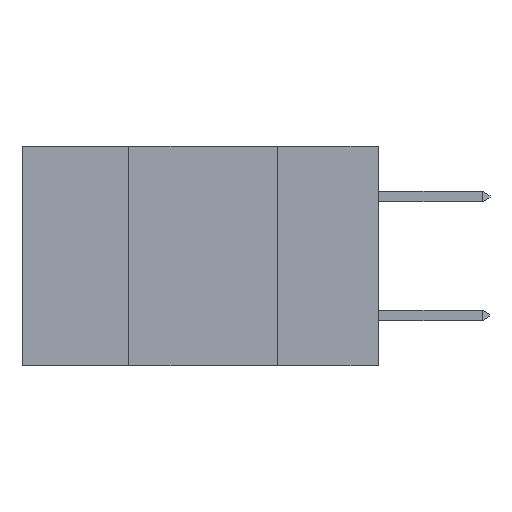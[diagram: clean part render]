
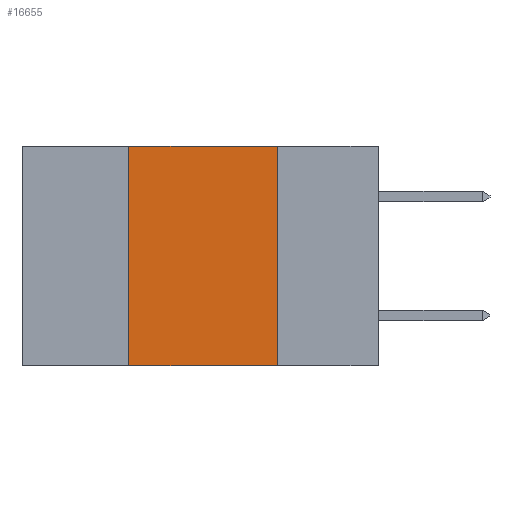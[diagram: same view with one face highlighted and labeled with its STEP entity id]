
A CAD part, left-side view. The second image highlights one B-rep face of the part: STEP entity #16655.
In plain terms, the highlighted planar face has unit normal (-1, 0, 0).
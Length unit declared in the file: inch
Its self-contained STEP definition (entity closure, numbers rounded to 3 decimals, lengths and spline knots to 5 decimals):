
#105 = CARTESIAN_POINT ( 'NONE',  ( 0., 0.17, -0.37 ) ) ;
#190 = AXIS2_PLACEMENT_3D ( 'NONE', #7293, #16573, #8641 ) ;
#1633 = CARTESIAN_POINT ( 'NONE',  ( 0., 0.6, -0.37 ) ) ;
#2129 = VECTOR ( 'NONE', #10610, 39.37008 ) ;
#3081 = DIRECTION ( 'NONE',  ( 0., -1., 0. ) ) ;
#3130 = EDGE_LOOP ( 'NONE', ( #14088, #11663, #10739, #10531 ) ) ;
#3622 = VECTOR ( 'NONE', #5970, 39.37008 ) ;
#5017 = EDGE_CURVE ( 'NONE', #16510, #5583, #6052, .T. ) ;
#5238 = CARTESIAN_POINT ( 'NONE',  ( 0., 0.17, 0. ) ) ;
#5350 = VERTEX_POINT ( 'NONE', #105 ) ;
#5583 = VERTEX_POINT ( 'NONE', #10946 ) ;
#5630 = LINE ( 'NONE', #5238, #2129 ) ;
#5970 = DIRECTION ( 'NONE',  ( 0., -1., 0. ) ) ;
#6052 = LINE ( 'NONE', #14876, #13534 ) ;
#6517 = VECTOR ( 'NONE', #3081, 39.37008 ) ;
#7272 = CARTESIAN_POINT ( 'NONE',  ( 0., 0.42, -0.37 ) ) ;
#7293 = CARTESIAN_POINT ( 'NONE',  ( 0., 0.6, 0. ) ) ;
#8641 = DIRECTION ( 'NONE',  ( 0., 0., -1. ) ) ;
#9177 = VERTEX_POINT ( 'NONE', #15960 ) ;
#9938 = PLANE ( 'NONE',  #190 ) ;
#10531 = ORIENTED_EDGE ( 'NONE', *, *, #13902, .T. ) ;
#10610 = DIRECTION ( 'NONE',  ( 0., 0., -1. ) ) ;
#10739 = ORIENTED_EDGE ( 'NONE', *, *, #5017, .F. ) ;
#10855 = FACE_OUTER_BOUND ( 'NONE', #3130, .T. ) ;
#10946 = CARTESIAN_POINT ( 'NONE',  ( 0., 0.42, 0. ) ) ;
#11663 = ORIENTED_EDGE ( 'NONE', *, *, #17330, .F. ) ;
#12619 = CARTESIAN_POINT ( 'NONE',  ( 0., 0.6, 0. ) ) ;
#13534 = VECTOR ( 'NONE', #15531, 39.37008 ) ;
#13902 = EDGE_CURVE ( 'NONE', #16510, #5350, #17086, .T. ) ;
#14088 = ORIENTED_EDGE ( 'NONE', *, *, #16336, .F. ) ;
#14114 = LINE ( 'NONE', #12619, #3622 ) ;
#14876 = CARTESIAN_POINT ( 'NONE',  ( 0., 0.42, 0. ) ) ;
#15531 = DIRECTION ( 'NONE',  ( 0., 0., 1. ) ) ;
#15960 = CARTESIAN_POINT ( 'NONE',  ( 0., 0.17, 0. ) ) ;
#16336 = EDGE_CURVE ( 'NONE', #9177, #5350, #5630, .T. ) ;
#16510 = VERTEX_POINT ( 'NONE', #7272 ) ;
#16573 = DIRECTION ( 'NONE',  ( 1., 0., 0. ) ) ;
#16655 = ADVANCED_FACE ( 'NONE', ( #10855 ), #9938, .F. ) ;
#17086 = LINE ( 'NONE', #1633, #6517 ) ;
#17330 = EDGE_CURVE ( 'NONE', #5583, #9177, #14114, .T. ) ;
